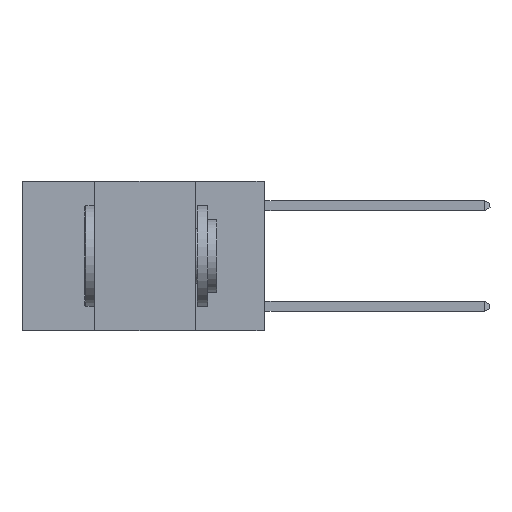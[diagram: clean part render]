
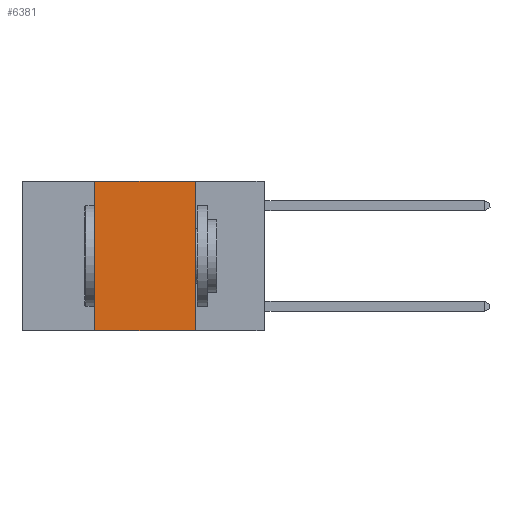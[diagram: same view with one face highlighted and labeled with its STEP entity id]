
A CAD part, left-side view. The second image highlights one B-rep face of the part: STEP entity #6381.
In plain terms, the highlighted planar face has unit normal (-1, 0, 0).
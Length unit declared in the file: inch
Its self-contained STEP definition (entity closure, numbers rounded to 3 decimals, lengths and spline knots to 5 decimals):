
#298 = VECTOR ( 'NONE', #2019, 39.37008 ) ;
#479 = CARTESIAN_POINT ( 'NONE',  ( 0., 0.6, 0. ) ) ;
#527 = FACE_OUTER_BOUND ( 'NONE', #1290, .T. ) ;
#655 = DIRECTION ( 'NONE',  ( 0., 0., -1. ) ) ;
#1165 = CARTESIAN_POINT ( 'NONE',  ( 0., 0.42, 0. ) ) ;
#1290 = EDGE_LOOP ( 'NONE', ( #1585, #2468, #6382, #4991 ) ) ;
#1334 = PLANE ( 'NONE',  #6511 ) ;
#1585 = ORIENTED_EDGE ( 'NONE', *, *, #6771, .F. ) ;
#1724 = CARTESIAN_POINT ( 'NONE',  ( 0., 0.17, 0. ) ) ;
#2019 = DIRECTION ( 'NONE',  ( 0., -1., 0. ) ) ;
#2468 = ORIENTED_EDGE ( 'NONE', *, *, #6265, .F. ) ;
#2587 = DIRECTION ( 'NONE',  ( 0., -1., 0. ) ) ;
#2666 = CARTESIAN_POINT ( 'NONE',  ( 0., 0.42, 0. ) ) ;
#2839 = LINE ( 'NONE', #1724, #8192 ) ;
#3075 = LINE ( 'NONE', #479, #6559 ) ;
#3403 = VERTEX_POINT ( 'NONE', #3962 ) ;
#3452 = CARTESIAN_POINT ( 'NONE',  ( 0., 0.17, 0. ) ) ;
#3839 = LINE ( 'NONE', #6193, #298 ) ;
#3962 = CARTESIAN_POINT ( 'NONE',  ( 0., 0.42, -0.37 ) ) ;
#4822 = CARTESIAN_POINT ( 'NONE',  ( 0., 0.17, -0.37 ) ) ;
#4862 = DIRECTION ( 'NONE',  ( 1., 0., 0. ) ) ;
#4991 = ORIENTED_EDGE ( 'NONE', *, *, #7589, .T. ) ;
#5063 = EDGE_CURVE ( 'NONE', #3403, #8876, #8573, .T. ) ;
#6049 = DIRECTION ( 'NONE',  ( 0., 0., 1. ) ) ;
#6193 = CARTESIAN_POINT ( 'NONE',  ( 0., 0.6, -0.37 ) ) ;
#6265 = EDGE_CURVE ( 'NONE', #8876, #6389, #3075, .T. ) ;
#6381 = ADVANCED_FACE ( 'NONE', ( #527 ), #1334, .F. ) ;
#6382 = ORIENTED_EDGE ( 'NONE', *, *, #5063, .F. ) ;
#6389 = VERTEX_POINT ( 'NONE', #3452 ) ;
#6511 = AXIS2_PLACEMENT_3D ( 'NONE', #7609, #4862, #655 ) ;
#6559 = VECTOR ( 'NONE', #2587, 39.37008 ) ;
#6771 = EDGE_CURVE ( 'NONE', #6389, #6942, #2839, .T. ) ;
#6942 = VERTEX_POINT ( 'NONE', #4822 ) ;
#7589 = EDGE_CURVE ( 'NONE', #3403, #6942, #3839, .T. ) ;
#7609 = CARTESIAN_POINT ( 'NONE',  ( 0., 0.6, 0. ) ) ;
#8037 = DIRECTION ( 'NONE',  ( 0., 0., -1. ) ) ;
#8158 = VECTOR ( 'NONE', #6049, 39.37008 ) ;
#8192 = VECTOR ( 'NONE', #8037, 39.37008 ) ;
#8573 = LINE ( 'NONE', #1165, #8158 ) ;
#8876 = VERTEX_POINT ( 'NONE', #2666 ) ;
